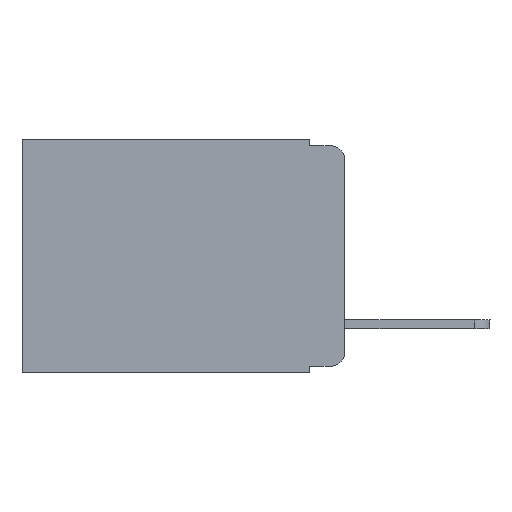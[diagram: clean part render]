
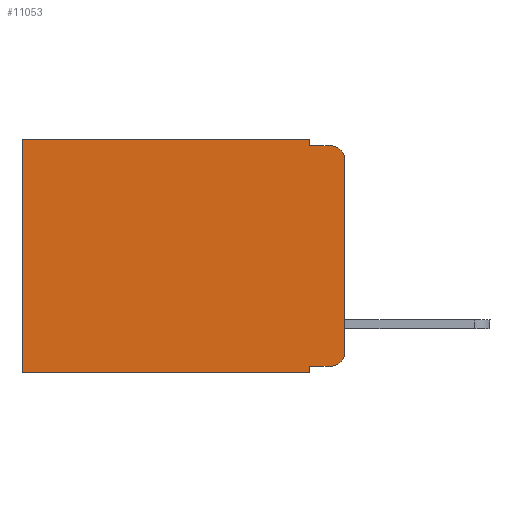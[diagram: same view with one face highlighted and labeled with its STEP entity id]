
A CAD part, left-side view. The second image highlights one B-rep face of the part: STEP entity #11053.
In plain terms, the highlighted planar face has unit normal (-1, 0, 0).
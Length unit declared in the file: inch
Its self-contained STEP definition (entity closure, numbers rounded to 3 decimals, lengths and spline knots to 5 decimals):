
#14 = ORIENTED_EDGE ( 'NONE', *, *, #9488, .F. ) ;
#230 = LINE ( 'NONE', #3198, #11723 ) ;
#486 = LINE ( 'NONE', #11042, #13761 ) ;
#666 = EDGE_CURVE ( 'NONE', #7090, #9748, #1154, .T. ) ;
#857 = ORIENTED_EDGE ( 'NONE', *, *, #3118, .T. ) ;
#866 = EDGE_CURVE ( 'NONE', #5306, #9748, #9532, .T. ) ;
#918 = DIRECTION ( 'NONE',  ( 0., 1., 0. ) ) ;
#985 = ORIENTED_EDGE ( 'NONE', *, *, #14848, .F. ) ;
#1154 = CIRCLE ( 'NONE', #3370, 0.02 ) ;
#1367 = EDGE_CURVE ( 'NONE', #5644, #15525, #1443, .T. ) ;
#1418 = CARTESIAN_POINT ( 'NONE',  ( 0.298, 0., -0.03 ) ) ;
#1443 = LINE ( 'NONE', #10488, #9402 ) ;
#1466 = EDGE_LOOP ( 'NONE', ( #3099, #857, #15094, #14303, #6594, #13305, #985, #14, #17025, #12740 ) ) ;
#1688 = CARTESIAN_POINT ( 'NONE',  ( 0.298, 0.02, -0.03 ) ) ;
#1797 = LINE ( 'NONE', #6876, #17010 ) ;
#2006 = VECTOR ( 'NONE', #10459, 39.37008 ) ;
#2484 = AXIS2_PLACEMENT_3D ( 'NONE', #14605, #17322, #6784 ) ;
#2761 = EDGE_CURVE ( 'NONE', #10646, #5644, #1797, .T. ) ;
#3099 = ORIENTED_EDGE ( 'NONE', *, *, #866, .F. ) ;
#3118 = EDGE_CURVE ( 'NONE', #5306, #15525, #15944, .T. ) ;
#3198 = CARTESIAN_POINT ( 'NONE',  ( 0.298, 0.051, 0. ) ) ;
#3206 = VECTOR ( 'NONE', #15163, 39.37008 ) ;
#3370 = AXIS2_PLACEMENT_3D ( 'NONE', #4412, #9813, #15145 ) ;
#3396 = CARTESIAN_POINT ( 'NONE',  ( 0.298, 0.051, -0.01 ) ) ;
#4160 = EDGE_CURVE ( 'NONE', #17130, #7090, #16476, .T. ) ;
#4412 = CARTESIAN_POINT ( 'NONE',  ( 0.298, 0.02, -0.313 ) ) ;
#5306 = VERTEX_POINT ( 'NONE', #1418 ) ;
#5443 = DIRECTION ( 'NONE',  ( 0., -1., 0. ) ) ;
#5644 = VERTEX_POINT ( 'NONE', #3396 ) ;
#5797 = CARTESIAN_POINT ( 'NONE',  ( 0.298, 0.473, 0. ) ) ;
#6266 = CARTESIAN_POINT ( 'NONE',  ( 0.298, 0.051, -0.343 ) ) ;
#6384 = EDGE_CURVE ( 'NONE', #13398, #16092, #486, .T. ) ;
#6577 = CARTESIAN_POINT ( 'NONE',  ( 0.298, 0.02, -0.333 ) ) ;
#6594 = ORIENTED_EDGE ( 'NONE', *, *, #13901, .T. ) ;
#6784 = DIRECTION ( 'NONE',  ( 0., 0., -1. ) ) ;
#6876 = CARTESIAN_POINT ( 'NONE',  ( 0.298, 0.051, 0. ) ) ;
#7090 = VERTEX_POINT ( 'NONE', #6577 ) ;
#7193 = CARTESIAN_POINT ( 'NONE',  ( 0.298, 0.051, -0.333 ) ) ;
#7200 = DIRECTION ( 'NONE',  ( -1., 0., 0. ) ) ;
#7475 = CARTESIAN_POINT ( 'NONE',  ( 0.298, 0., 0. ) ) ;
#8287 = CARTESIAN_POINT ( 'NONE',  ( 0.298, 0.473, -0.343 ) ) ;
#9402 = VECTOR ( 'NONE', #5443, 39.37008 ) ;
#9488 = EDGE_CURVE ( 'NONE', #17130, #14138, #230, .T. ) ;
#9532 = LINE ( 'NONE', #14875, #12688 ) ;
#9748 = VERTEX_POINT ( 'NONE', #16090 ) ;
#9813 = DIRECTION ( 'NONE',  ( -1., 0., 0. ) ) ;
#10459 = DIRECTION ( 'NONE',  ( 0., 1., 0. ) ) ;
#10488 = CARTESIAN_POINT ( 'NONE',  ( 0.298, 0.051, -0.01 ) ) ;
#10646 = VERTEX_POINT ( 'NONE', #17205 ) ;
#10863 = DIRECTION ( 'NONE',  ( 0., 0., -1. ) ) ;
#11042 = CARTESIAN_POINT ( 'NONE',  ( 0.298, 0.473, 0. ) ) ;
#11053 = ADVANCED_FACE ( 'NONE', ( #13107 ), #16174, .F. ) ;
#11321 = CARTESIAN_POINT ( 'NONE',  ( 0.298, 0.02, -0.01 ) ) ;
#11626 = CARTESIAN_POINT ( 'NONE',  ( 0.298, 0., -0.343 ) ) ;
#11723 = VECTOR ( 'NONE', #13827, 39.37008 ) ;
#12243 = DIRECTION ( 'NONE',  ( 0., 0., -1. ) ) ;
#12300 = AXIS2_PLACEMENT_3D ( 'NONE', #1688, #7200, #12549 ) ;
#12549 = DIRECTION ( 'NONE',  ( 0., 0., -1. ) ) ;
#12688 = VECTOR ( 'NONE', #10863, 39.37008 ) ;
#12740 = ORIENTED_EDGE ( 'NONE', *, *, #666, .T. ) ;
#12926 = LINE ( 'NONE', #11626, #14362 ) ;
#13107 = FACE_OUTER_BOUND ( 'NONE', #1466, .T. ) ;
#13305 = ORIENTED_EDGE ( 'NONE', *, *, #6384, .T. ) ;
#13398 = VERTEX_POINT ( 'NONE', #5797 ) ;
#13761 = VECTOR ( 'NONE', #12243, 39.37008 ) ;
#13827 = DIRECTION ( 'NONE',  ( 0., 0., -1. ) ) ;
#13901 = EDGE_CURVE ( 'NONE', #10646, #13398, #16855, .T. ) ;
#14138 = VERTEX_POINT ( 'NONE', #6266 ) ;
#14303 = ORIENTED_EDGE ( 'NONE', *, *, #2761, .F. ) ;
#14362 = VECTOR ( 'NONE', #918, 39.37008 ) ;
#14605 = CARTESIAN_POINT ( 'NONE',  ( 0.298, 0., 0. ) ) ;
#14848 = EDGE_CURVE ( 'NONE', #14138, #16092, #12926, .T. ) ;
#14875 = CARTESIAN_POINT ( 'NONE',  ( 0.298, 0., 0. ) ) ;
#14946 = DIRECTION ( 'NONE',  ( 0., 0., -1. ) ) ;
#15094 = ORIENTED_EDGE ( 'NONE', *, *, #1367, .F. ) ;
#15145 = DIRECTION ( 'NONE',  ( 0., 0., -1. ) ) ;
#15163 = DIRECTION ( 'NONE',  ( 0., -1., 0. ) ) ;
#15525 = VERTEX_POINT ( 'NONE', #11321 ) ;
#15944 = CIRCLE ( 'NONE', #12300, 0.02 ) ;
#16090 = CARTESIAN_POINT ( 'NONE',  ( 0.298, 0., -0.313 ) ) ;
#16092 = VERTEX_POINT ( 'NONE', #8287 ) ;
#16174 = PLANE ( 'NONE',  #2484 ) ;
#16476 = LINE ( 'NONE', #7193, #3206 ) ;
#16855 = LINE ( 'NONE', #7475, #2006 ) ;
#16871 = CARTESIAN_POINT ( 'NONE',  ( 0.298, 0.051, -0.333 ) ) ;
#17010 = VECTOR ( 'NONE', #14946, 39.37008 ) ;
#17025 = ORIENTED_EDGE ( 'NONE', *, *, #4160, .T. ) ;
#17130 = VERTEX_POINT ( 'NONE', #16871 ) ;
#17205 = CARTESIAN_POINT ( 'NONE',  ( 0.298, 0.051, 0. ) ) ;
#17322 = DIRECTION ( 'NONE',  ( 1., 0., 0. ) ) ;
